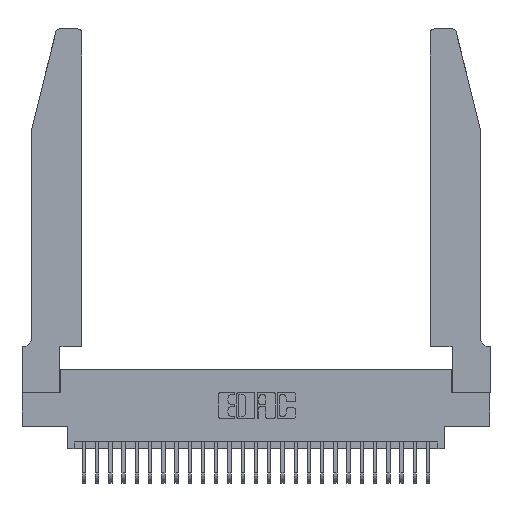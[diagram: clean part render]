
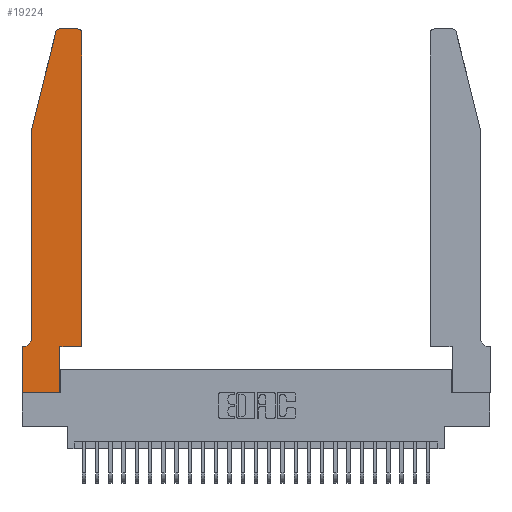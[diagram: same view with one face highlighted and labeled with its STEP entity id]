
A CAD part, top view. The second image highlights one B-rep face of the part: STEP entity #19224.
In plain terms, the highlighted planar face has unit normal (0, 0, 1).
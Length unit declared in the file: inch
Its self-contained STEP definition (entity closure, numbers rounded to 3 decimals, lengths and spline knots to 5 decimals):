
#313 = CARTESIAN_POINT ( 'NONE',  ( 0.0755, 2., 0.37 ) ) ;
#326 = VECTOR ( 'NONE', #12945, 39.37008 ) ;
#359 = EDGE_CURVE ( 'NONE', #1962, #2886, #28541, .T. ) ;
#409 = DIRECTION ( 'NONE',  ( 1., 0., 0. ) ) ;
#428 = VERTEX_POINT ( 'NONE', #993 ) ;
#772 = LINE ( 'NONE', #29740, #23049 ) ;
#993 = CARTESIAN_POINT ( 'NONE',  ( 0.4505, 2.72, 0.37 ) ) ;
#1177 = CARTESIAN_POINT ( 'NONE',  ( 0.284, 2.72, 0.37 ) ) ;
#1461 = LINE ( 'NONE', #22377, #13172 ) ;
#1506 = ORIENTED_EDGE ( 'NONE', *, *, #359, .T. ) ;
#1658 = AXIS2_PLACEMENT_3D ( 'NONE', #14189, #14155, #13926 ) ;
#1962 = VERTEX_POINT ( 'NONE', #18668 ) ;
#2198 = EDGE_CURVE ( 'NONE', #3362, #11137, #19969, .T. ) ;
#2886 = VERTEX_POINT ( 'NONE', #19415 ) ;
#3362 = VERTEX_POINT ( 'NONE', #11734 ) ;
#3580 = DIRECTION ( 'NONE',  ( 1., 0., 0. ) ) ;
#3658 = CIRCLE ( 'NONE', #13127, 0.03 ) ;
#4287 = DIRECTION ( 'NONE',  ( 1., 0., 0. ) ) ;
#4466 = EDGE_CURVE ( 'NONE', #6169, #1962, #22988, .T. ) ;
#4705 = DIRECTION ( 'NONE',  ( -1., 0., 0. ) ) ;
#4953 = CARTESIAN_POINT ( 'NONE',  ( 0., 0., 0.37 ) ) ;
#5065 = LINE ( 'NONE', #8551, #27868 ) ;
#5384 = CARTESIAN_POINT ( 'NONE',  ( 0.2865, 0., 0.37 ) ) ;
#5700 = CARTESIAN_POINT ( 'NONE',  ( 0.25487, 2.72718, 0.37 ) ) ;
#5718 = CARTESIAN_POINT ( 'NONE',  ( 0.4505, 0.35, 0.37 ) ) ;
#5798 = AXIS2_PLACEMENT_3D ( 'NONE', #11995, #27803, #14286 ) ;
#6026 = FACE_OUTER_BOUND ( 'NONE', #16660, .T. ) ;
#6169 = VERTEX_POINT ( 'NONE', #13247 ) ;
#6668 = LINE ( 'NONE', #8739, #12835 ) ;
#7808 = LINE ( 'NONE', #313, #13921 ) ;
#8551 = CARTESIAN_POINT ( 'NONE',  ( 0.2605, 2.75, 0.37 ) ) ;
#8739 = CARTESIAN_POINT ( 'NONE',  ( 0., 0., 0.37 ) ) ;
#8910 = ORIENTED_EDGE ( 'NONE', *, *, #16048, .T. ) ;
#9101 = CARTESIAN_POINT ( 'NONE',  ( 0., 0., 0.37 ) ) ;
#9278 = ORIENTED_EDGE ( 'NONE', *, *, #15182, .T. ) ;
#10612 = CARTESIAN_POINT ( 'NONE',  ( 0.2865, 0.35, 0.37 ) ) ;
#10848 = DIRECTION ( 'NONE',  ( -1., 0., 0. ) ) ;
#10934 = DIRECTION ( 'NONE',  ( 0., -1., 0. ) ) ;
#11137 = VERTEX_POINT ( 'NONE', #18356 ) ;
#11397 = ORIENTED_EDGE ( 'NONE', *, *, #15632, .T. ) ;
#11716 = VECTOR ( 'NONE', #27487, 39.37008 ) ;
#11734 = CARTESIAN_POINT ( 'NONE',  ( 0.2865, 0.35, 0.37 ) ) ;
#11754 = ORIENTED_EDGE ( 'NONE', *, *, #27635, .T. ) ;
#11995 = CARTESIAN_POINT ( 'NONE',  ( 0., 0.35, 0.37 ) ) ;
#12175 = AXIS2_PLACEMENT_3D ( 'NONE', #1177, #17394, #3580 ) ;
#12835 = VECTOR ( 'NONE', #10934, 39.37008 ) ;
#12872 = EDGE_CURVE ( 'NONE', #27874, #14907, #16160, .T. ) ;
#12945 = DIRECTION ( 'NONE',  ( 0., 1., 0. ) ) ;
#13127 = AXIS2_PLACEMENT_3D ( 'NONE', #27912, #14396, #409 ) ;
#13172 = VECTOR ( 'NONE', #24628, 39.37008 ) ;
#13247 = CARTESIAN_POINT ( 'NONE',  ( 0.0755, 2., 0.37 ) ) ;
#13571 = ORIENTED_EDGE ( 'NONE', *, *, #20709, .T. ) ;
#13690 = CARTESIAN_POINT ( 'NONE',  ( 0.4205, 2.75, 0.37 ) ) ;
#13796 = VERTEX_POINT ( 'NONE', #15134 ) ;
#13921 = VECTOR ( 'NONE', #25514, 39.37008 ) ;
#13926 = DIRECTION ( 'NONE',  ( -1., 0., 0. ) ) ;
#13976 = CARTESIAN_POINT ( 'NONE',  ( 0.0755, 2., 0.37 ) ) ;
#14155 = DIRECTION ( 'NONE',  ( 0., 0., -1. ) ) ;
#14189 = CARTESIAN_POINT ( 'NONE',  ( 0.0055, 0.42, 0.37 ) ) ;
#14286 = DIRECTION ( 'NONE',  ( 1., 0., 0. ) ) ;
#14396 = DIRECTION ( 'NONE',  ( 0., 0., 1. ) ) ;
#14907 = VERTEX_POINT ( 'NONE', #5384 ) ;
#15134 = CARTESIAN_POINT ( 'NONE',  ( 0., 0.35, 0.37 ) ) ;
#15182 = EDGE_CURVE ( 'NONE', #13796, #27874, #6668, .T. ) ;
#15632 = EDGE_CURVE ( 'NONE', #14907, #3362, #18827, .T. ) ;
#16048 = EDGE_CURVE ( 'NONE', #428, #29061, #3658, .T. ) ;
#16160 = LINE ( 'NONE', #9101, #17570 ) ;
#16660 = EDGE_LOOP ( 'NONE', ( #17099, #29112, #11754, #19231, #1506, #19925, #9278, #27313, #11397, #18888, #13571, #8910 ) ) ;
#17099 = ORIENTED_EDGE ( 'NONE', *, *, #18122, .T. ) ;
#17394 = DIRECTION ( 'NONE',  ( 0., 0., 1. ) ) ;
#17570 = VECTOR ( 'NONE', #4287, 39.37008 ) ;
#18002 = VERTEX_POINT ( 'NONE', #5700 ) ;
#18122 = EDGE_CURVE ( 'NONE', #29061, #27262, #5065, .T. ) ;
#18356 = CARTESIAN_POINT ( 'NONE',  ( 0.4505, 0.35, 0.37 ) ) ;
#18562 = VECTOR ( 'NONE', #19444, 39.37008 ) ;
#18668 = CARTESIAN_POINT ( 'NONE',  ( 0.0755, 0.42, 0.37 ) ) ;
#18827 = LINE ( 'NONE', #10612, #326 ) ;
#18888 = ORIENTED_EDGE ( 'NONE', *, *, #2198, .T. ) ;
#19224 = ADVANCED_FACE ( 'NONE', ( #6026 ), #25506, .T. ) ;
#19231 = ORIENTED_EDGE ( 'NONE', *, *, #4466, .T. ) ;
#19415 = CARTESIAN_POINT ( 'NONE',  ( 0.0055, 0.35, 0.37 ) ) ;
#19444 = DIRECTION ( 'NONE',  ( 1., 0., 0. ) ) ;
#19580 = CARTESIAN_POINT ( 'NONE',  ( 0.284, 2.75, 0.37 ) ) ;
#19925 = ORIENTED_EDGE ( 'NONE', *, *, #28480, .T. ) ;
#19969 = LINE ( 'NONE', #5718, #18562 ) ;
#20709 = EDGE_CURVE ( 'NONE', #11137, #428, #1461, .T. ) ;
#22377 = CARTESIAN_POINT ( 'NONE',  ( 0.4505, 0.35, 0.37 ) ) ;
#22988 = LINE ( 'NONE', #13976, #11716 ) ;
#23049 = VECTOR ( 'NONE', #4705, 39.37008 ) ;
#24628 = DIRECTION ( 'NONE',  ( 0., 1., 0. ) ) ;
#25506 = PLANE ( 'NONE',  #5798 ) ;
#25514 = DIRECTION ( 'NONE',  ( -0.239, -0.971, 0. ) ) ;
#25563 = CIRCLE ( 'NONE', #12175, 0.03 ) ;
#27262 = VERTEX_POINT ( 'NONE', #19580 ) ;
#27313 = ORIENTED_EDGE ( 'NONE', *, *, #12872, .T. ) ;
#27487 = DIRECTION ( 'NONE',  ( 0., -1., 0. ) ) ;
#27635 = EDGE_CURVE ( 'NONE', #18002, #6169, #7808, .T. ) ;
#27803 = DIRECTION ( 'NONE',  ( 0., 0., 1. ) ) ;
#27868 = VECTOR ( 'NONE', #10848, 39.37008 ) ;
#27874 = VERTEX_POINT ( 'NONE', #4953 ) ;
#27912 = CARTESIAN_POINT ( 'NONE',  ( 0.4205, 2.72, 0.37 ) ) ;
#28143 = EDGE_CURVE ( 'NONE', #27262, #18002, #25563, .T. ) ;
#28480 = EDGE_CURVE ( 'NONE', #2886, #13796, #772, .T. ) ;
#28541 = CIRCLE ( 'NONE', #1658, 0.07 ) ;
#29061 = VERTEX_POINT ( 'NONE', #13690 ) ;
#29112 = ORIENTED_EDGE ( 'NONE', *, *, #28143, .T. ) ;
#29740 = CARTESIAN_POINT ( 'NONE',  ( 0.0755, 0.35, 0.37 ) ) ;
